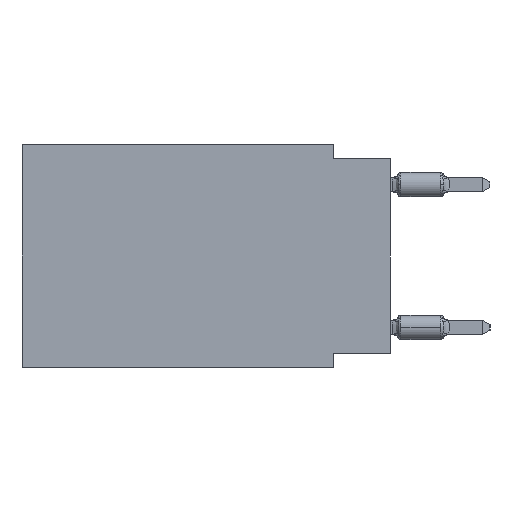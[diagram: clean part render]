
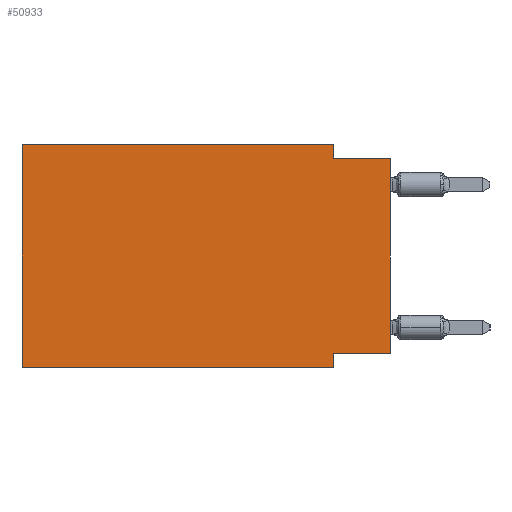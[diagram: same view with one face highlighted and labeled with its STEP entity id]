
A CAD part, left-side view. The second image highlights one B-rep face of the part: STEP entity #50933.
In plain terms, the highlighted planar face has unit normal (-1, 0, 0).
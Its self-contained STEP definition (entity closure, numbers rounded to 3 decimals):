
#1029 = DIRECTION ( 'NONE',  ( 0., -1., 0. ) ) ;
#1181 = CARTESIAN_POINT ( 'NONE',  ( 0., 0., -9.271 ) ) ;
#2565 = VERTEX_POINT ( 'NONE', #35098 ) ;
#2849 = CARTESIAN_POINT ( 'NONE',  ( 0., 2.54, 0. ) ) ;
#3061 = DIRECTION ( 'NONE',  ( 1., 0., 0. ) ) ;
#4659 = LINE ( 'NONE', #39275, #42492 ) ;
#6173 = CARTESIAN_POINT ( 'NONE',  ( 0., 16.383, -9.906 ) ) ;
#6992 = CARTESIAN_POINT ( 'NONE',  ( 0., 16.383, 0. ) ) ;
#7051 = LINE ( 'NONE', #24047, #38685 ) ;
#7913 = VERTEX_POINT ( 'NONE', #52559 ) ;
#9606 = CARTESIAN_POINT ( 'NONE',  ( 0., 16.383, 0. ) ) ;
#9735 = LINE ( 'NONE', #39584, #29382 ) ;
#10221 = VECTOR ( 'NONE', #53087, 1000. ) ;
#10479 = CARTESIAN_POINT ( 'NONE',  ( 0., 2.54, -9.906 ) ) ;
#11622 = CARTESIAN_POINT ( 'NONE',  ( 0., 16.383, -9.906 ) ) ;
#12270 = VECTOR ( 'NONE', #35752, 1000. ) ;
#13259 = VECTOR ( 'NONE', #18443, 1000. ) ;
#13613 = CARTESIAN_POINT ( 'NONE',  ( 0., 0., -0.635 ) ) ;
#14343 = EDGE_LOOP ( 'NONE', ( #38387, #47968, #34628, #32659, #36972, #48941, #41538, #34971 ) ) ;
#17375 = VERTEX_POINT ( 'NONE', #2849 ) ;
#18090 = DIRECTION ( 'NONE',  ( 0., 0., -1. ) ) ;
#18443 = DIRECTION ( 'NONE',  ( 0., -1., 0. ) ) ;
#19530 = VERTEX_POINT ( 'NONE', #47974 ) ;
#19862 = DIRECTION ( 'NONE',  ( 0., 0., 1. ) ) ;
#20337 = EDGE_CURVE ( 'NONE', #7913, #17375, #27097, .T. ) ;
#23940 = VECTOR ( 'NONE', #43090, 1000. ) ;
#24047 = CARTESIAN_POINT ( 'NONE',  ( 0., 0., 0. ) ) ;
#25242 = EDGE_CURVE ( 'NONE', #42730, #7913, #48385, .T. ) ;
#27085 = CARTESIAN_POINT ( 'NONE',  ( 0., 0., -9.271 ) ) ;
#27097 = LINE ( 'NONE', #48611, #10221 ) ;
#29382 = VECTOR ( 'NONE', #18090, 1000. ) ;
#32659 = ORIENTED_EDGE ( 'NONE', *, *, #20337, .F. ) ;
#32930 = DIRECTION ( 'NONE',  ( 0., 0., -1. ) ) ;
#34262 = EDGE_CURVE ( 'NONE', #49267, #19530, #39660, .T. ) ;
#34628 = ORIENTED_EDGE ( 'NONE', *, *, #38757, .F. ) ;
#34971 = ORIENTED_EDGE ( 'NONE', *, *, #34262, .F. ) ;
#35098 = CARTESIAN_POINT ( 'NONE',  ( 0., 2.54, -9.906 ) ) ;
#35581 = EDGE_CURVE ( 'NONE', #42730, #2565, #44410, .T. ) ;
#35752 = DIRECTION ( 'NONE',  ( 0., 1., 0. ) ) ;
#36434 = DIRECTION ( 'NONE',  ( 0., 0., -1. ) ) ;
#36571 = PLANE ( 'NONE',  #42219 ) ;
#36972 = ORIENTED_EDGE ( 'NONE', *, *, #25242, .F. ) ;
#38387 = ORIENTED_EDGE ( 'NONE', *, *, #49418, .T. ) ;
#38512 = VERTEX_POINT ( 'NONE', #53627 ) ;
#38685 = VECTOR ( 'NONE', #19862, 1000. ) ;
#38757 = EDGE_CURVE ( 'NONE', #17375, #38512, #9735, .T. ) ;
#39275 = CARTESIAN_POINT ( 'NONE',  ( 0., 0., -0.635 ) ) ;
#39584 = CARTESIAN_POINT ( 'NONE',  ( 0., 2.54, 0. ) ) ;
#39660 = LINE ( 'NONE', #27085, #12270 ) ;
#41166 = LINE ( 'NONE', #10479, #43799 ) ;
#41538 = ORIENTED_EDGE ( 'NONE', *, *, #47736, .F. ) ;
#42219 = AXIS2_PLACEMENT_3D ( 'NONE', #6992, #3061, #32930 ) ;
#42468 = EDGE_CURVE ( 'NONE', #38512, #43743, #4659, .T. ) ;
#42492 = VECTOR ( 'NONE', #1029, 1000. ) ;
#42730 = VERTEX_POINT ( 'NONE', #11622 ) ;
#43090 = DIRECTION ( 'NONE',  ( 0., 0., 1. ) ) ;
#43618 = FACE_OUTER_BOUND ( 'NONE', #14343, .T. ) ;
#43743 = VERTEX_POINT ( 'NONE', #13613 ) ;
#43799 = VECTOR ( 'NONE', #36434, 1000. ) ;
#44410 = LINE ( 'NONE', #6173, #13259 ) ;
#47736 = EDGE_CURVE ( 'NONE', #19530, #2565, #41166, .T. ) ;
#47968 = ORIENTED_EDGE ( 'NONE', *, *, #42468, .F. ) ;
#47974 = CARTESIAN_POINT ( 'NONE',  ( 0., 2.54, -9.271 ) ) ;
#48385 = LINE ( 'NONE', #9606, #23940 ) ;
#48611 = CARTESIAN_POINT ( 'NONE',  ( 0., 16.383, 0. ) ) ;
#48941 = ORIENTED_EDGE ( 'NONE', *, *, #35581, .T. ) ;
#49267 = VERTEX_POINT ( 'NONE', #1181 ) ;
#49418 = EDGE_CURVE ( 'NONE', #49267, #43743, #7051, .T. ) ;
#50933 = ADVANCED_FACE ( 'NONE', ( #43618 ), #36571, .F. ) ;
#52559 = CARTESIAN_POINT ( 'NONE',  ( 0., 16.383, 0. ) ) ;
#53087 = DIRECTION ( 'NONE',  ( 0., -1., 0. ) ) ;
#53627 = CARTESIAN_POINT ( 'NONE',  ( 0., 2.54, -0.635 ) ) ;
